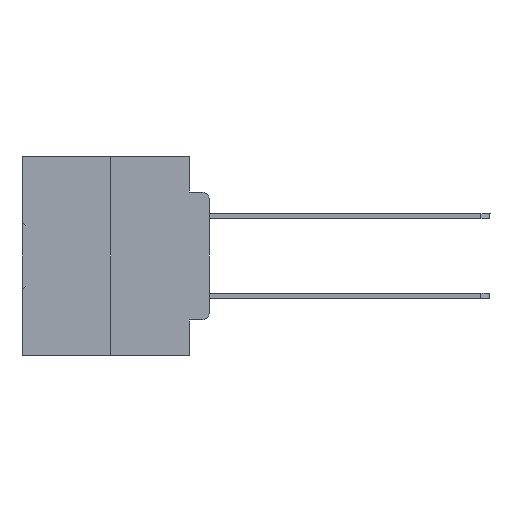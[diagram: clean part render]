
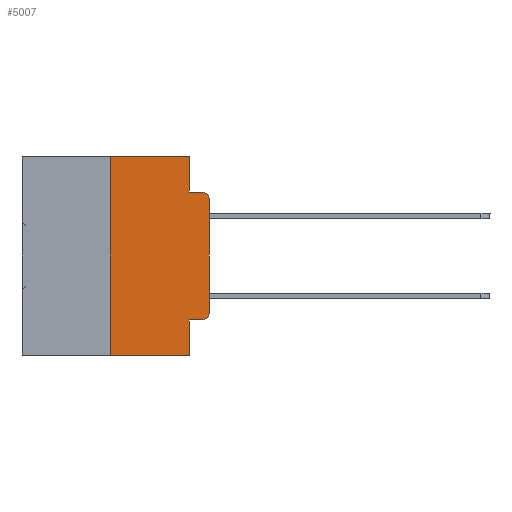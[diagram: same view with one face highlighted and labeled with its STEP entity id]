
A CAD part, left-side view. The second image highlights one B-rep face of the part: STEP entity #5007.
In plain terms, the highlighted planar face has unit normal (-1, 0, 0).
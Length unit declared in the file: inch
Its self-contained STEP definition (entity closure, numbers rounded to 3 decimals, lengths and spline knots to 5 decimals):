
#302 = CARTESIAN_POINT ( 'NONE',  ( 0., 0.02, -0.3915 ) ) ;
#1214 = DIRECTION ( 'NONE',  ( 0., 0., 1. ) ) ;
#1215 = ORIENTED_EDGE ( 'NONE', *, *, #31735, .T. ) ;
#1921 = ORIENTED_EDGE ( 'NONE', *, *, #8830, .F. ) ;
#3116 = DIRECTION ( 'NONE',  ( 0., -1., 0. ) ) ;
#3156 = VERTEX_POINT ( 'NONE', #17705 ) ;
#3220 = EDGE_CURVE ( 'NONE', #16075, #15151, #22906, .T. ) ;
#3267 = CARTESIAN_POINT ( 'NONE',  ( 0., 0.473, 0. ) ) ;
#3965 = DIRECTION ( 'NONE',  ( 0., -1., 0. ) ) ;
#3969 = CARTESIAN_POINT ( 'NONE',  ( 0., 0.25, 0. ) ) ;
#4516 = CARTESIAN_POINT ( 'NONE',  ( 0., 0.051, 0. ) ) ;
#4920 = CARTESIAN_POINT ( 'NONE',  ( 0., 0., 0. ) ) ;
#5007 = ADVANCED_FACE ( 'NONE', ( #20253 ), #20627, .F. ) ;
#5021 = CARTESIAN_POINT ( 'NONE',  ( 0., 0.051, -0.4115 ) ) ;
#5326 = VECTOR ( 'NONE', #30449, 39.37008 ) ;
#5736 = EDGE_CURVE ( 'NONE', #16075, #36565, #24126, .T. ) ;
#5836 = CARTESIAN_POINT ( 'NONE',  ( 0., 0.473, 0. ) ) ;
#5852 = CARTESIAN_POINT ( 'NONE',  ( 0., 0.051, -0.0885 ) ) ;
#6547 = VECTOR ( 'NONE', #16571, 39.37008 ) ;
#6713 = EDGE_LOOP ( 'NONE', ( #1215, #16941, #30617, #11804, #23753, #1921, #29377, #34318, #34866, #16538 ) ) ;
#8203 = DIRECTION ( 'NONE',  ( 0., 0., -1. ) ) ;
#8380 = DIRECTION ( 'NONE',  ( -1., 0., 0. ) ) ;
#8830 = EDGE_CURVE ( 'NONE', #13525, #3156, #32100, .T. ) ;
#8973 = AXIS2_PLACEMENT_3D ( 'NONE', #17073, #8380, #8203 ) ;
#8990 = AXIS2_PLACEMENT_3D ( 'NONE', #3267, #14728, #23587 ) ;
#11252 = VECTOR ( 'NONE', #28909, 39.37008 ) ;
#11804 = ORIENTED_EDGE ( 'NONE', *, *, #31126, .F. ) ;
#12141 = VECTOR ( 'NONE', #14172, 39.37008 ) ;
#12313 = CARTESIAN_POINT ( 'NONE',  ( 0., 0.051, -0.5 ) ) ;
#13525 = VERTEX_POINT ( 'NONE', #28080 ) ;
#13648 = AXIS2_PLACEMENT_3D ( 'NONE', #302, #28416, #25266 ) ;
#13831 = CARTESIAN_POINT ( 'NONE',  ( 0., 0.051, 0. ) ) ;
#14172 = DIRECTION ( 'NONE',  ( 0., -1., 0. ) ) ;
#14728 = DIRECTION ( 'NONE',  ( 1., 0., 0. ) ) ;
#14893 = LINE ( 'NONE', #29505, #25165 ) ;
#15151 = VERTEX_POINT ( 'NONE', #27742 ) ;
#15369 = VERTEX_POINT ( 'NONE', #13831 ) ;
#15542 = VECTOR ( 'NONE', #35451, 39.37008 ) ;
#15842 = LINE ( 'NONE', #4920, #6547 ) ;
#16075 = VERTEX_POINT ( 'NONE', #5021 ) ;
#16538 = ORIENTED_EDGE ( 'NONE', *, *, #31852, .T. ) ;
#16571 = DIRECTION ( 'NONE',  ( 0., 0., 1. ) ) ;
#16941 = ORIENTED_EDGE ( 'NONE', *, *, #23718, .T. ) ;
#17073 = CARTESIAN_POINT ( 'NONE',  ( 0., 0.02, -0.1085 ) ) ;
#17420 = CARTESIAN_POINT ( 'NONE',  ( 0., 0., -0.3915 ) ) ;
#17705 = CARTESIAN_POINT ( 'NONE',  ( 0., 0.25, 0. ) ) ;
#18456 = CARTESIAN_POINT ( 'NONE',  ( 0., 0.02, -0.0885 ) ) ;
#20177 = CIRCLE ( 'NONE', #8973, 0.02 ) ;
#20253 = FACE_OUTER_BOUND ( 'NONE', #6713, .T. ) ;
#20627 = PLANE ( 'NONE',  #8990 ) ;
#21434 = EDGE_CURVE ( 'NONE', #3156, #15369, #28052, .T. ) ;
#22725 = VERTEX_POINT ( 'NONE', #18456 ) ;
#22764 = CARTESIAN_POINT ( 'NONE',  ( 0., 0.051, -0.0885 ) ) ;
#22906 = LINE ( 'NONE', #34771, #27560 ) ;
#23587 = DIRECTION ( 'NONE',  ( 0., 0., -1. ) ) ;
#23718 = EDGE_CURVE ( 'NONE', #28929, #22725, #20177, .T. ) ;
#23753 = ORIENTED_EDGE ( 'NONE', *, *, #21434, .F. ) ;
#24126 = LINE ( 'NONE', #4516, #15542 ) ;
#24534 = EDGE_CURVE ( 'NONE', #25689, #22725, #34178, .T. ) ;
#24727 = EDGE_CURVE ( 'NONE', #13525, #36565, #14893, .T. ) ;
#25165 = VECTOR ( 'NONE', #3965, 39.37008 ) ;
#25266 = DIRECTION ( 'NONE',  ( 0., 0., -1. ) ) ;
#25689 = VERTEX_POINT ( 'NONE', #22764 ) ;
#27560 = VECTOR ( 'NONE', #3116, 39.37008 ) ;
#27742 = CARTESIAN_POINT ( 'NONE',  ( 0., 0.02, -0.4115 ) ) ;
#28052 = LINE ( 'NONE', #5836, #5326 ) ;
#28080 = CARTESIAN_POINT ( 'NONE',  ( 0., 0.25, -0.5 ) ) ;
#28416 = DIRECTION ( 'NONE',  ( -1., 0., 0. ) ) ;
#28909 = DIRECTION ( 'NONE',  ( 0., 0., -1. ) ) ;
#28929 = VERTEX_POINT ( 'NONE', #36179 ) ;
#29377 = ORIENTED_EDGE ( 'NONE', *, *, #24727, .T. ) ;
#29505 = CARTESIAN_POINT ( 'NONE',  ( 0., 0.473, -0.5 ) ) ;
#29573 = LINE ( 'NONE', #29747, #11252 ) ;
#29610 = CIRCLE ( 'NONE', #13648, 0.02 ) ;
#29747 = CARTESIAN_POINT ( 'NONE',  ( 0., 0.051, 0. ) ) ;
#30449 = DIRECTION ( 'NONE',  ( 0., -1., 0. ) ) ;
#30617 = ORIENTED_EDGE ( 'NONE', *, *, #24534, .F. ) ;
#30696 = VECTOR ( 'NONE', #1214, 39.37008 ) ;
#31126 = EDGE_CURVE ( 'NONE', #15369, #25689, #29573, .T. ) ;
#31735 = EDGE_CURVE ( 'NONE', #35473, #28929, #15842, .T. ) ;
#31852 = EDGE_CURVE ( 'NONE', #15151, #35473, #29610, .T. ) ;
#32100 = LINE ( 'NONE', #3969, #30696 ) ;
#34178 = LINE ( 'NONE', #5852, #12141 ) ;
#34318 = ORIENTED_EDGE ( 'NONE', *, *, #5736, .F. ) ;
#34771 = CARTESIAN_POINT ( 'NONE',  ( 0., 0.051, -0.4115 ) ) ;
#34866 = ORIENTED_EDGE ( 'NONE', *, *, #3220, .T. ) ;
#35451 = DIRECTION ( 'NONE',  ( 0., 0., -1. ) ) ;
#35473 = VERTEX_POINT ( 'NONE', #17420 ) ;
#36179 = CARTESIAN_POINT ( 'NONE',  ( 0., 0., -0.1085 ) ) ;
#36565 = VERTEX_POINT ( 'NONE', #12313 ) ;
